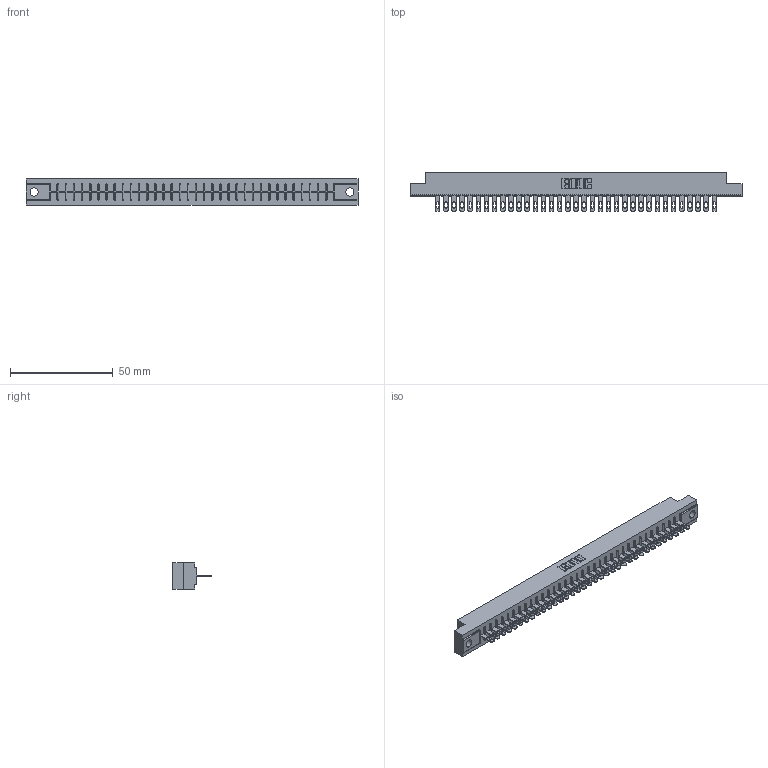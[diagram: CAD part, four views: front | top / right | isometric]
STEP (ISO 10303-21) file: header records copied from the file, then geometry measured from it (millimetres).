
FILE_DESCRIPTION (( 'STEP AP203' ), '1' );
FILE_NAME ('356-035-500-104.STEP', '2018-08-01T21:40:25', ( '' ), ( '' ), 'SwSTEP 2.0', 'SolidWorks 2016', '' );
FILE_SCHEMA (( 'CONFIG_CONTROL_DESIGN' ));
Length unit declared in the file: inch
Products named in the file (3): 356-035-500-104; 306 Part_.156 Dia; 306-290-001_100
Assembly tree (36 placements, depth 2):
  356-035-500-104
    306 Part_.156 Dia
    306-290-001_100  x35
Bounding box: 161.7 x 18.87 x 12.7 mm (x, y, z)
Volume: 17823 mm3; surface area: 18654.5 mm2
Topology: 36 solids, 36 shells, 2790 faces, 7877 edges, 5062 vertices
Faces by surface type: plane 1832, cylinder 818, sphere 140
Entity records: 34128 total; most frequent: CARTESIAN_POINT 5734, ORIENTED_EDGE 5682, DIRECTION 5647, EDGE_CURVE 2841, VECTOR 2225, LINE 2225, VERTEX_POINT 1798, AXIS2_PLACEMENT_3D 1711
